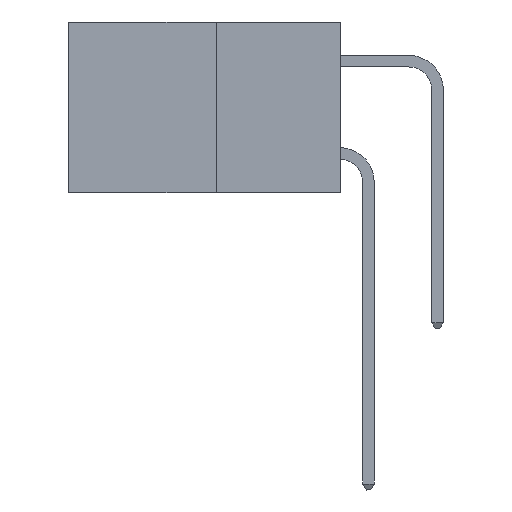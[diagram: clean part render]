
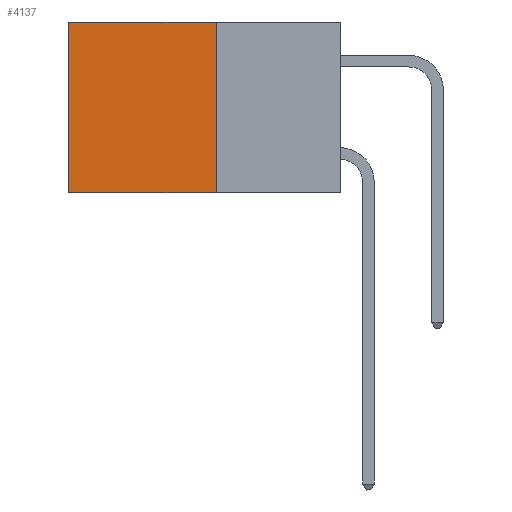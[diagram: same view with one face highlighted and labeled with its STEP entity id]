
A CAD part, left-side view. The second image highlights one B-rep face of the part: STEP entity #4137.
In plain terms, the highlighted planar face has unit normal (-1, 0, 0).
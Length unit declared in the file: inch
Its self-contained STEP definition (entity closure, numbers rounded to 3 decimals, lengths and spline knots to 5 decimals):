
#288 = EDGE_LOOP ( 'NONE', ( #20947, #14352, #6753, #6327 ) ) ;
#1108 = VECTOR ( 'NONE', #21955, 39.37008 ) ;
#1214 = VERTEX_POINT ( 'NONE', #25137 ) ;
#2132 = PLANE ( 'NONE',  #20867 ) ;
#3109 = EDGE_CURVE ( 'NONE', #1214, #22463, #6984, .T. ) ;
#4137 = ADVANCED_FACE ( 'NONE', ( #6563 ), #2132, .F. ) ;
#6327 = ORIENTED_EDGE ( 'NONE', *, *, #13707, .T. ) ;
#6563 = FACE_OUTER_BOUND ( 'NONE', #288, .T. ) ;
#6753 = ORIENTED_EDGE ( 'NONE', *, *, #10006, .F. ) ;
#6984 = LINE ( 'NONE', #19099, #1108 ) ;
#7194 = DIRECTION ( 'NONE',  ( 0., 0., -1. ) ) ;
#7310 = DIRECTION ( 'NONE',  ( 1., 0., 0. ) ) ;
#7382 = DIRECTION ( 'NONE',  ( 0., 0., -1. ) ) ;
#7468 = CARTESIAN_POINT ( 'NONE',  ( 0.277, 0.27, -0.37 ) ) ;
#7713 = VECTOR ( 'NONE', #7792, 39.37008 ) ;
#7792 = DIRECTION ( 'NONE',  ( 0., 1., 0. ) ) ;
#8380 = CARTESIAN_POINT ( 'NONE',  ( 0.277, 0.27, -0.37 ) ) ;
#10006 = EDGE_CURVE ( 'NONE', #24818, #1214, #22340, .T. ) ;
#10802 = CARTESIAN_POINT ( 'NONE',  ( 0.277, 0.59, -0.37 ) ) ;
#11520 = CARTESIAN_POINT ( 'NONE',  ( 0.277, 0.59, 0. ) ) ;
#13197 = EDGE_CURVE ( 'NONE', #19211, #22463, #20145, .T. ) ;
#13669 = CARTESIAN_POINT ( 'NONE',  ( 0.277, 0.27, 0. ) ) ;
#13707 = EDGE_CURVE ( 'NONE', #24818, #19211, #18748, .T. ) ;
#14314 = VECTOR ( 'NONE', #7382, 39.37008 ) ;
#14352 = ORIENTED_EDGE ( 'NONE', *, *, #3109, .F. ) ;
#16544 = VECTOR ( 'NONE', #19459, 39.37008 ) ;
#18365 = CARTESIAN_POINT ( 'NONE',  ( 0.277, 0.59, -0.37 ) ) ;
#18748 = LINE ( 'NONE', #25320, #7713 ) ;
#19099 = CARTESIAN_POINT ( 'NONE',  ( 0.277, 0.27, -0.37 ) ) ;
#19211 = VERTEX_POINT ( 'NONE', #11520 ) ;
#19459 = DIRECTION ( 'NONE',  ( 0., 0., -1. ) ) ;
#20145 = LINE ( 'NONE', #18365, #14314 ) ;
#20867 = AXIS2_PLACEMENT_3D ( 'NONE', #7468, #7310, #7194 ) ;
#20947 = ORIENTED_EDGE ( 'NONE', *, *, #13197, .T. ) ;
#21955 = DIRECTION ( 'NONE',  ( 0., 1., 0. ) ) ;
#22340 = LINE ( 'NONE', #8380, #16544 ) ;
#22463 = VERTEX_POINT ( 'NONE', #10802 ) ;
#24818 = VERTEX_POINT ( 'NONE', #13669 ) ;
#25137 = CARTESIAN_POINT ( 'NONE',  ( 0.277, 0.27, -0.37 ) ) ;
#25320 = CARTESIAN_POINT ( 'NONE',  ( 0.277, 0.27, 0. ) ) ;
